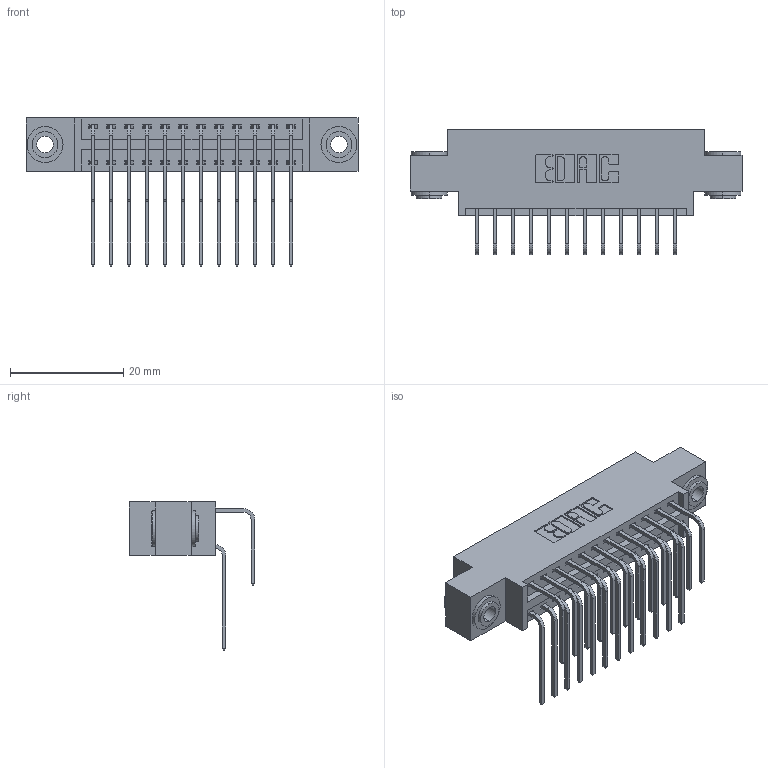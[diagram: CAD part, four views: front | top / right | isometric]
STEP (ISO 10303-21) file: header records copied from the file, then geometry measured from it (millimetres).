
FILE_DESCRIPTION (( 'STEP AP203' ), '1' );
FILE_NAME ('346-024-558-803.STEP', '2022-05-19T00:19:58', ( '' ), ( '' ), 'SwSTEP 2.0', 'SolidWorks 2020', '' );
FILE_SCHEMA (( 'CONFIG_CONTROL_DESIGN' ));
Length unit declared in the file: inch
Products named in the file (5): 345-292-001_558 559 Tail - 1; 346 Part_0.170 Offset - 0.156 Dia-TH; 345-250-002_345-250-002-102; 345-292-001_558 Tail - 2; 346-024-558-803
Assembly tree (27 placements, depth 2):
  346-024-558-803
    346 Part_0.170 Offset - 0.156 Dia-TH
    345-292-001_558 559 Tail - 1  x12
    345-292-001_558 Tail - 2  x12
    345-250-002_345-250-002-102  x2
Bounding box: 58.67 x 22.16 x 26.16 mm (x, y, z)
Volume: 5473.6 mm3; surface area: 8144.8 mm2
Topology: 27 solids, 27 shells, 1474 faces, 4317 edges, 2842 vertices
Faces by surface type: plane 992, cylinder 474, cone 8
Entity records: 14852 total; most frequent: CARTESIAN_POINT 2524, ORIENTED_EDGE 2398, DIRECTION 2277, EDGE_CURVE 1199, VECTOR 955, LINE 955, VERTEX_POINT 794, AXIS2_PLACEMENT_3D 661
